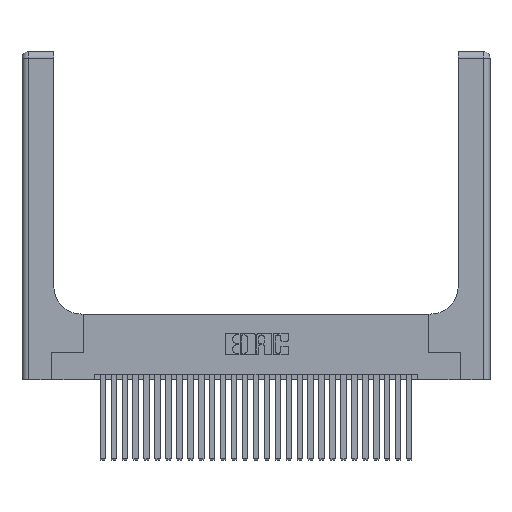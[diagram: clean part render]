
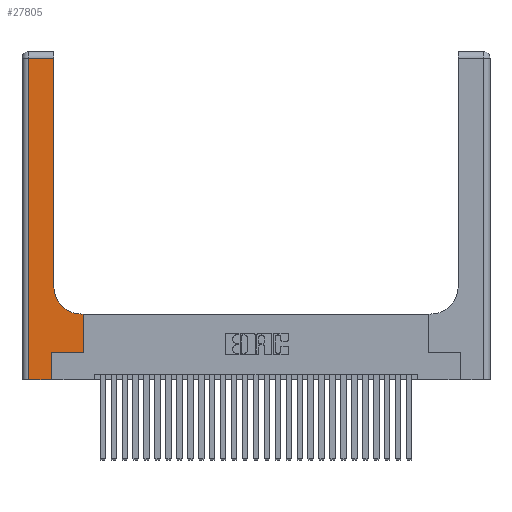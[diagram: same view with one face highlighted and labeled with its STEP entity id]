
A CAD part, top view. The second image highlights one B-rep face of the part: STEP entity #27805.
In plain terms, the highlighted planar face has unit normal (0, 0, 1).
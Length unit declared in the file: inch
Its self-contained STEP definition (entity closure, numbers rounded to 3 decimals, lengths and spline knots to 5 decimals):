
#212 = CARTESIAN_POINT ( 'NONE',  ( 0.5415, 0.6, 0.37 ) ) ;
#1135 = VECTOR ( 'NONE', #14972, 39.37008 ) ;
#1288 = VERTEX_POINT ( 'NONE', #212 ) ;
#1322 = PLANE ( 'NONE',  #17177 ) ;
#1547 = LINE ( 'NONE', #7913, #4382 ) ;
#2646 = VERTEX_POINT ( 'NONE', #9382 ) ;
#2725 = CARTESIAN_POINT ( 'NONE',  ( 0.5585, 0.25, 0.37 ) ) ;
#4136 = EDGE_CURVE ( 'NONE', #12915, #16911, #9728, .T. ) ;
#4226 = EDGE_LOOP ( 'NONE', ( #11262, #19997, #12799, #20285, #24479, #17278, #12454, #25021, #17302 ) ) ;
#4382 = VECTOR ( 'NONE', #24175, 39.37008 ) ;
#5775 = DIRECTION ( 'NONE',  ( 0., 1., 0. ) ) ;
#5941 = CARTESIAN_POINT ( 'NONE',  ( 0.5585, 0.6, 0.37 ) ) ;
#6457 = LINE ( 'NONE', #6697, #8161 ) ;
#6638 = LINE ( 'NONE', #24034, #27311 ) ;
#6697 = CARTESIAN_POINT ( 'NONE',  ( 0.5585, 0.25, 0.37 ) ) ;
#7108 = VERTEX_POINT ( 'NONE', #17351 ) ;
#7129 = LINE ( 'NONE', #15427, #27489 ) ;
#7913 = CARTESIAN_POINT ( 'NONE',  ( 0.269, 0.25, 0.37 ) ) ;
#8161 = VECTOR ( 'NONE', #22469, 39.37008 ) ;
#8278 = VERTEX_POINT ( 'NONE', #5941 ) ;
#8554 = DIRECTION ( 'NONE',  ( 0., 1., 0. ) ) ;
#8776 = DIRECTION ( 'NONE',  ( 0., 0., -1. ) ) ;
#8954 = EDGE_CURVE ( 'NONE', #7108, #22984, #1547, .T. ) ;
#9382 = CARTESIAN_POINT ( 'NONE',  ( 0.2915, 2.94, 0.37 ) ) ;
#9728 = LINE ( 'NONE', #10904, #21184 ) ;
#10314 = CARTESIAN_POINT ( 'NONE',  ( 0., 3., 0.37 ) ) ;
#10487 = EDGE_CURVE ( 'NONE', #16911, #7108, #7129, .T. ) ;
#10701 = CARTESIAN_POINT ( 'NONE',  ( 0.06, 2.94, 0.37 ) ) ;
#10904 = CARTESIAN_POINT ( 'NONE',  ( 0., 0., 0.37 ) ) ;
#11262 = ORIENTED_EDGE ( 'NONE', *, *, #27766, .T. ) ;
#12326 = CIRCLE ( 'NONE', #12621, 0.25 ) ;
#12454 = ORIENTED_EDGE ( 'NONE', *, *, #24514, .T. ) ;
#12621 = AXIS2_PLACEMENT_3D ( 'NONE', #20488, #8776, #16059 ) ;
#12799 = ORIENTED_EDGE ( 'NONE', *, *, #19723, .T. ) ;
#12915 = VERTEX_POINT ( 'NONE', #21952 ) ;
#14972 = DIRECTION ( 'NONE',  ( 0., -1., 0. ) ) ;
#15010 = DIRECTION ( 'NONE',  ( -1., 0., 0. ) ) ;
#15427 = CARTESIAN_POINT ( 'NONE',  ( 0.269, 0., 0.37 ) ) ;
#16059 = DIRECTION ( 'NONE',  ( 1., 0., 0. ) ) ;
#16911 = VERTEX_POINT ( 'NONE', #27831 ) ;
#17064 = CARTESIAN_POINT ( 'NONE',  ( 0.06, 3., 0.37 ) ) ;
#17177 = AXIS2_PLACEMENT_3D ( 'NONE', #10314, #17204, #24224 ) ;
#17204 = DIRECTION ( 'NONE',  ( 0., 0., -1. ) ) ;
#17278 = ORIENTED_EDGE ( 'NONE', *, *, #8954, .T. ) ;
#17302 = ORIENTED_EDGE ( 'NONE', *, *, #27298, .T. ) ;
#17351 = CARTESIAN_POINT ( 'NONE',  ( 0.269, 0.25, 0.37 ) ) ;
#17380 = CARTESIAN_POINT ( 'NONE',  ( 0.2915, 0.6, 0.37 ) ) ;
#18030 = FACE_OUTER_BOUND ( 'NONE', #4226, .T. ) ;
#19723 = EDGE_CURVE ( 'NONE', #28576, #12915, #26814, .T. ) ;
#19997 = ORIENTED_EDGE ( 'NONE', *, *, #23040, .T. ) ;
#20285 = ORIENTED_EDGE ( 'NONE', *, *, #4136, .T. ) ;
#20488 = CARTESIAN_POINT ( 'NONE',  ( 0.5415, 0.85, 0.37 ) ) ;
#20899 = VECTOR ( 'NONE', #21043, 39.37008 ) ;
#21043 = DIRECTION ( 'NONE',  ( -1., 0., 0. ) ) ;
#21184 = VECTOR ( 'NONE', #29200, 39.37008 ) ;
#21422 = EDGE_CURVE ( 'NONE', #8278, #1288, #23517, .T. ) ;
#21952 = CARTESIAN_POINT ( 'NONE',  ( 0.06, 0., 0.37 ) ) ;
#22455 = VECTOR ( 'NONE', #15010, 39.37008 ) ;
#22469 = DIRECTION ( 'NONE',  ( 0., 1., 0. ) ) ;
#22784 = VERTEX_POINT ( 'NONE', #29461 ) ;
#22984 = VERTEX_POINT ( 'NONE', #2725 ) ;
#23040 = EDGE_CURVE ( 'NONE', #2646, #28576, #26988, .T. ) ;
#23517 = LINE ( 'NONE', #17380, #22455 ) ;
#23547 = CARTESIAN_POINT ( 'NONE',  ( 0., 2.94, 0.37 ) ) ;
#24034 = CARTESIAN_POINT ( 'NONE',  ( 0.2915, 3., 0.37 ) ) ;
#24175 = DIRECTION ( 'NONE',  ( 1., 0., 0. ) ) ;
#24224 = DIRECTION ( 'NONE',  ( -1., 0., 0. ) ) ;
#24479 = ORIENTED_EDGE ( 'NONE', *, *, #10487, .T. ) ;
#24514 = EDGE_CURVE ( 'NONE', #22984, #8278, #6457, .T. ) ;
#25021 = ORIENTED_EDGE ( 'NONE', *, *, #21422, .T. ) ;
#26814 = LINE ( 'NONE', #17064, #1135 ) ;
#26988 = LINE ( 'NONE', #23547, #20899 ) ;
#27298 = EDGE_CURVE ( 'NONE', #1288, #22784, #12326, .T. ) ;
#27311 = VECTOR ( 'NONE', #5775, 39.37008 ) ;
#27489 = VECTOR ( 'NONE', #8554, 39.37008 ) ;
#27766 = EDGE_CURVE ( 'NONE', #22784, #2646, #6638, .T. ) ;
#27805 = ADVANCED_FACE ( 'NONE', ( #18030 ), #1322, .F. ) ;
#27831 = CARTESIAN_POINT ( 'NONE',  ( 0.269, 0., 0.37 ) ) ;
#28576 = VERTEX_POINT ( 'NONE', #10701 ) ;
#29200 = DIRECTION ( 'NONE',  ( 1., 0., 0. ) ) ;
#29461 = CARTESIAN_POINT ( 'NONE',  ( 0.2915, 0.85, 0.37 ) ) ;
